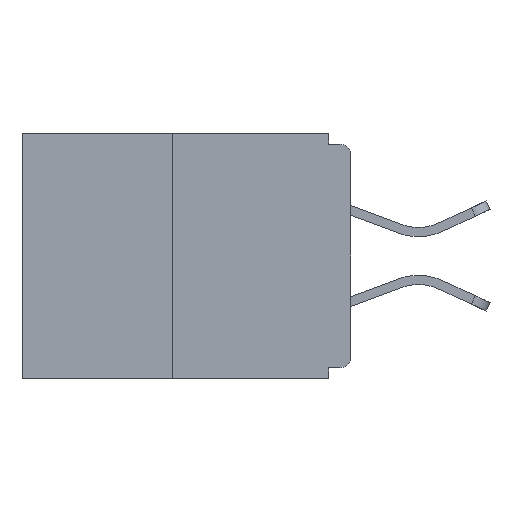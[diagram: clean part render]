
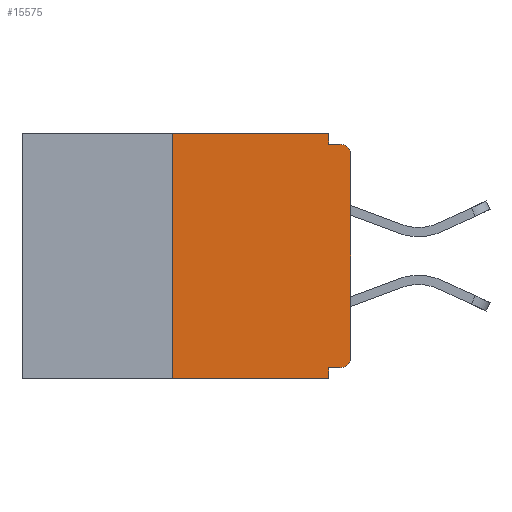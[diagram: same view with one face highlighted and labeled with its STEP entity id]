
A CAD part, left-side view. The second image highlights one B-rep face of the part: STEP entity #15575.
In plain terms, the highlighted planar face has unit normal (-1, 0, 0).
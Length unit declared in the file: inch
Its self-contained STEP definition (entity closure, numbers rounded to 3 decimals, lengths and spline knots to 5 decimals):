
#250 = CARTESIAN_POINT ( 'NONE',  ( 0., 0.031, -0.015 ) ) ;
#256 = ORIENTED_EDGE ( 'NONE', *, *, #420, .F. ) ;
#420 = EDGE_CURVE ( 'NONE', #12662, #11382, #12761, .T. ) ;
#477 = VERTEX_POINT ( 'NONE', #3134 ) ;
#521 = DIRECTION ( 'NONE',  ( -1., 0., 0. ) ) ;
#1350 = FACE_OUTER_BOUND ( 'NONE', #16052, .T. ) ;
#1355 = ORIENTED_EDGE ( 'NONE', *, *, #10627, .F. ) ;
#1551 = LINE ( 'NONE', #5937, #13723 ) ;
#1553 = VECTOR ( 'NONE', #14170, 39.37008 ) ;
#1754 = CARTESIAN_POINT ( 'NONE',  ( 0., 0.015, -0.328 ) ) ;
#1892 = VECTOR ( 'NONE', #6299, 39.37008 ) ;
#1953 = DIRECTION ( 'NONE',  ( 0., 0., 1. ) ) ;
#2155 = CARTESIAN_POINT ( 'NONE',  ( 0., 0.25, 0. ) ) ;
#2215 = CARTESIAN_POINT ( 'NONE',  ( 0., 0.015, -0.313 ) ) ;
#2288 = DIRECTION ( 'NONE',  ( 0., 0., -1. ) ) ;
#2819 = EDGE_CURVE ( 'NONE', #11382, #13740, #1551, .T. ) ;
#3084 = VECTOR ( 'NONE', #7993, 39.37008 ) ;
#3134 = CARTESIAN_POINT ( 'NONE',  ( 0., 0.031, 0. ) ) ;
#3553 = ORIENTED_EDGE ( 'NONE', *, *, #5224, .F. ) ;
#3794 = AXIS2_PLACEMENT_3D ( 'NONE', #18551, #18264, #13392 ) ;
#4191 = CARTESIAN_POINT ( 'NONE',  ( 0., 0.015, -0.03 ) ) ;
#4365 = AXIS2_PLACEMENT_3D ( 'NONE', #2215, #13750, #2288 ) ;
#4763 = LINE ( 'NONE', #19636, #19191 ) ;
#5224 = EDGE_CURVE ( 'NONE', #9065, #14476, #19283, .T. ) ;
#5323 = EDGE_CURVE ( 'NONE', #7240, #13740, #18023, .T. ) ;
#5748 = CIRCLE ( 'NONE', #18168, 0.015 ) ;
#5937 = CARTESIAN_POINT ( 'NONE',  ( 0., 0.031, -0.343 ) ) ;
#6031 = EDGE_CURVE ( 'NONE', #20106, #7299, #18240, .T. ) ;
#6235 = ORIENTED_EDGE ( 'NONE', *, *, #15217, .F. ) ;
#6248 = CARTESIAN_POINT ( 'NONE',  ( 0., 0.031, -0.343 ) ) ;
#6299 = DIRECTION ( 'NONE',  ( 0., 1., 0. ) ) ;
#6461 = CARTESIAN_POINT ( 'NONE',  ( 0., 0.46, 0. ) ) ;
#6509 = ORIENTED_EDGE ( 'NONE', *, *, #6031, .T. ) ;
#7018 = ORIENTED_EDGE ( 'NONE', *, *, #5323, .T. ) ;
#7240 = VERTEX_POINT ( 'NONE', #13354 ) ;
#7299 = VERTEX_POINT ( 'NONE', #15514 ) ;
#7927 = VECTOR ( 'NONE', #10728, 39.37008 ) ;
#7993 = DIRECTION ( 'NONE',  ( 0., -1., 0. ) ) ;
#8979 = CIRCLE ( 'NONE', #4365, 0.015 ) ;
#9065 = VERTEX_POINT ( 'NONE', #250 ) ;
#9200 = EDGE_CURVE ( 'NONE', #12662, #20106, #8979, .T. ) ;
#9728 = CARTESIAN_POINT ( 'NONE',  ( 0., 0., 0. ) ) ;
#10627 = EDGE_CURVE ( 'NONE', #10711, #477, #20021, .T. ) ;
#10711 = VERTEX_POINT ( 'NONE', #2155 ) ;
#10728 = DIRECTION ( 'NONE',  ( 0., 0., -1. ) ) ;
#10820 = DIRECTION ( 'NONE',  ( 0., 0., -1. ) ) ;
#11102 = CARTESIAN_POINT ( 'NONE',  ( 0., 0., -0.015 ) ) ;
#11382 = VERTEX_POINT ( 'NONE', #16909 ) ;
#12662 = VERTEX_POINT ( 'NONE', #1754 ) ;
#12737 = ORIENTED_EDGE ( 'NONE', *, *, #2819, .F. ) ;
#12761 = LINE ( 'NONE', #14460, #1892 ) ;
#13354 = CARTESIAN_POINT ( 'NONE',  ( 0., 0.25, -0.343 ) ) ;
#13392 = DIRECTION ( 'NONE',  ( 0., 0., -1. ) ) ;
#13723 = VECTOR ( 'NONE', #10820, 39.37008 ) ;
#13740 = VERTEX_POINT ( 'NONE', #6248 ) ;
#13750 = DIRECTION ( 'NONE',  ( -1., 0., 0. ) ) ;
#13945 = VECTOR ( 'NONE', #16740, 39.37008 ) ;
#14170 = DIRECTION ( 'NONE',  ( 0., -1., 0. ) ) ;
#14460 = CARTESIAN_POINT ( 'NONE',  ( 0., 0., -0.328 ) ) ;
#14476 = VERTEX_POINT ( 'NONE', #15022 ) ;
#15022 = CARTESIAN_POINT ( 'NONE',  ( 0., 0.015, -0.015 ) ) ;
#15028 = LINE ( 'NONE', #15833, #7927 ) ;
#15217 = EDGE_CURVE ( 'NONE', #477, #9065, #15028, .T. ) ;
#15514 = CARTESIAN_POINT ( 'NONE',  ( 0., 0., -0.03 ) ) ;
#15575 = ADVANCED_FACE ( 'NONE', ( #1350 ), #16900, .F. ) ;
#15687 = VECTOR ( 'NONE', #19364, 39.37008 ) ;
#15833 = CARTESIAN_POINT ( 'NONE',  ( 0., 0.031, 0. ) ) ;
#16052 = EDGE_LOOP ( 'NONE', ( #1355, #16399, #7018, #12737, #256, #20449, #6509, #17348, #3553, #6235 ) ) ;
#16399 = ORIENTED_EDGE ( 'NONE', *, *, #19310, .F. ) ;
#16740 = DIRECTION ( 'NONE',  ( 0., 0., 1. ) ) ;
#16900 = PLANE ( 'NONE',  #3794 ) ;
#16909 = CARTESIAN_POINT ( 'NONE',  ( 0., 0.031, -0.328 ) ) ;
#17348 = ORIENTED_EDGE ( 'NONE', *, *, #18436, .T. ) ;
#17420 = CARTESIAN_POINT ( 'NONE',  ( 0., 0.46, -0.343 ) ) ;
#18023 = LINE ( 'NONE', #17420, #3084 ) ;
#18168 = AXIS2_PLACEMENT_3D ( 'NONE', #4191, #521, #18733 ) ;
#18240 = LINE ( 'NONE', #9728, #13945 ) ;
#18264 = DIRECTION ( 'NONE',  ( 1., 0., 0. ) ) ;
#18436 = EDGE_CURVE ( 'NONE', #7299, #14476, #5748, .T. ) ;
#18551 = CARTESIAN_POINT ( 'NONE',  ( 0., 0.46, 0. ) ) ;
#18733 = DIRECTION ( 'NONE',  ( 0., 0., -1. ) ) ;
#19191 = VECTOR ( 'NONE', #1953, 39.37008 ) ;
#19283 = LINE ( 'NONE', #11102, #1553 ) ;
#19310 = EDGE_CURVE ( 'NONE', #7240, #10711, #4763, .T. ) ;
#19364 = DIRECTION ( 'NONE',  ( 0., -1., 0. ) ) ;
#19636 = CARTESIAN_POINT ( 'NONE',  ( 0., 0.25, 0. ) ) ;
#20021 = LINE ( 'NONE', #6461, #15687 ) ;
#20106 = VERTEX_POINT ( 'NONE', #20557 ) ;
#20449 = ORIENTED_EDGE ( 'NONE', *, *, #9200, .T. ) ;
#20557 = CARTESIAN_POINT ( 'NONE',  ( 0., 0., -0.313 ) ) ;
